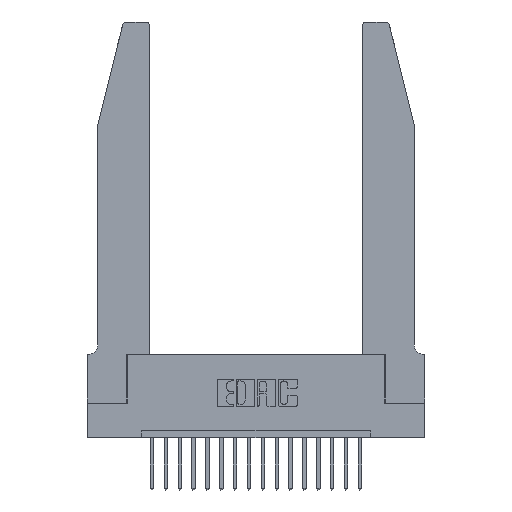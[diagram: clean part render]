
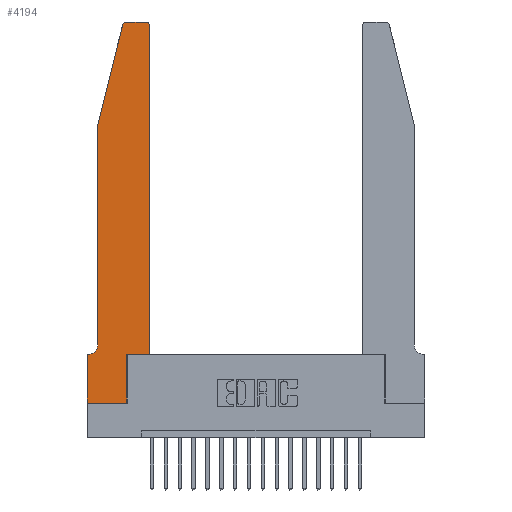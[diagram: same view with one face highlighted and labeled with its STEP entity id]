
A CAD part, top view. The second image highlights one B-rep face of the part: STEP entity #4194.
In plain terms, the highlighted planar face has unit normal (0, 0, 1).
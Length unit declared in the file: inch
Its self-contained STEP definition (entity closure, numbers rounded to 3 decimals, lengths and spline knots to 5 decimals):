
#94 = VERTEX_POINT ( 'NONE', #13322 ) ;
#170 = VERTEX_POINT ( 'NONE', #18015 ) ;
#202 = EDGE_CURVE ( 'NONE', #3944, #170, #8114, .T. ) ;
#376 = DIRECTION ( 'NONE',  ( 1., 0., 0. ) ) ;
#534 = EDGE_CURVE ( 'NONE', #94, #1270, #5633, .T. ) ;
#641 = CARTESIAN_POINT ( 'NONE',  ( 0.2605, 2.75, 0.37 ) ) ;
#1007 = DIRECTION ( 'NONE',  ( -1., 0., 0. ) ) ;
#1154 = CARTESIAN_POINT ( 'NONE',  ( 0.0055, 0.42, 0.37 ) ) ;
#1270 = VERTEX_POINT ( 'NONE', #15781 ) ;
#1276 = CARTESIAN_POINT ( 'NONE',  ( 0., 0.35, 0.37 ) ) ;
#1709 = VECTOR ( 'NONE', #8410, 39.37008 ) ;
#2233 = VERTEX_POINT ( 'NONE', #10709 ) ;
#2391 = ORIENTED_EDGE ( 'NONE', *, *, #17332, .T. ) ;
#2839 = DIRECTION ( 'NONE',  ( 1., 0., 0. ) ) ;
#2897 = DIRECTION ( 'NONE',  ( 0., -1., 0. ) ) ;
#2994 = VERTEX_POINT ( 'NONE', #13306 ) ;
#3384 = VECTOR ( 'NONE', #2897, 39.37008 ) ;
#3480 = CARTESIAN_POINT ( 'NONE',  ( 0., 0., 0.37 ) ) ;
#3659 = CARTESIAN_POINT ( 'NONE',  ( 0.4505, 0.35, 0.37 ) ) ;
#3829 = DIRECTION ( 'NONE',  ( -1., 0., 0. ) ) ;
#3839 = DIRECTION ( 'NONE',  ( -0.239, -0.971, 0. ) ) ;
#3944 = VERTEX_POINT ( 'NONE', #16292 ) ;
#4049 = FACE_OUTER_BOUND ( 'NONE', #19425, .T. ) ;
#4194 = ADVANCED_FACE ( 'NONE', ( #4049 ), #17205, .T. ) ;
#4573 = VERTEX_POINT ( 'NONE', #1276 ) ;
#4658 = LINE ( 'NONE', #12014, #15701 ) ;
#4729 = ORIENTED_EDGE ( 'NONE', *, *, #11184, .T. ) ;
#4768 = ORIENTED_EDGE ( 'NONE', *, *, #5936, .T. ) ;
#4908 = VECTOR ( 'NONE', #3839, 39.37008 ) ;
#5247 = ORIENTED_EDGE ( 'NONE', *, *, #202, .T. ) ;
#5402 = DIRECTION ( 'NONE',  ( -1., 0., 0. ) ) ;
#5448 = AXIS2_PLACEMENT_3D ( 'NONE', #1154, #12026, #1007 ) ;
#5456 = CARTESIAN_POINT ( 'NONE',  ( 0.4505, 0.35, 0.37 ) ) ;
#5633 = CIRCLE ( 'NONE', #6486, 0.03 ) ;
#5805 = ORIENTED_EDGE ( 'NONE', *, *, #534, .T. ) ;
#5936 = EDGE_CURVE ( 'NONE', #16654, #6398, #16736, .T. ) ;
#6065 = CARTESIAN_POINT ( 'NONE',  ( 0.0755, 2., 0.37 ) ) ;
#6201 = ORIENTED_EDGE ( 'NONE', *, *, #19285, .T. ) ;
#6398 = VERTEX_POINT ( 'NONE', #19903 ) ;
#6486 = AXIS2_PLACEMENT_3D ( 'NONE', #19861, #7242, #10382 ) ;
#6542 = AXIS2_PLACEMENT_3D ( 'NONE', #12942, #14470, #376 ) ;
#6652 = LINE ( 'NONE', #13153, #4908 ) ;
#7002 = LINE ( 'NONE', #641, #7955 ) ;
#7242 = DIRECTION ( 'NONE',  ( 0., 0., 1. ) ) ;
#7265 = ORIENTED_EDGE ( 'NONE', *, *, #16557, .T. ) ;
#7582 = LINE ( 'NONE', #11657, #16384 ) ;
#7955 = VECTOR ( 'NONE', #5402, 39.37008 ) ;
#8114 = LINE ( 'NONE', #18491, #17631 ) ;
#8335 = DIRECTION ( 'NONE',  ( 0., 1., 0. ) ) ;
#8339 = ORIENTED_EDGE ( 'NONE', *, *, #18361, .T. ) ;
#8410 = DIRECTION ( 'NONE',  ( 1., 0., 0. ) ) ;
#9039 = LINE ( 'NONE', #6065, #3384 ) ;
#9347 = DIRECTION ( 'NONE',  ( 0., 0., 1. ) ) ;
#9499 = VERTEX_POINT ( 'NONE', #18136 ) ;
#10382 = DIRECTION ( 'NONE',  ( 1., 0., 0. ) ) ;
#10709 = CARTESIAN_POINT ( 'NONE',  ( 0.284, 2.75, 0.37 ) ) ;
#11184 = EDGE_CURVE ( 'NONE', #2994, #9499, #6652, .T. ) ;
#11384 = ORIENTED_EDGE ( 'NONE', *, *, #15175, .T. ) ;
#11543 = LINE ( 'NONE', #3480, #12003 ) ;
#11635 = CARTESIAN_POINT ( 'NONE',  ( 0.0755, 0.42, 0.37 ) ) ;
#11657 = CARTESIAN_POINT ( 'NONE',  ( 0.0755, 0.35, 0.37 ) ) ;
#11877 = ORIENTED_EDGE ( 'NONE', *, *, #19243, .T. ) ;
#12003 = VECTOR ( 'NONE', #18964, 39.37008 ) ;
#12014 = CARTESIAN_POINT ( 'NONE',  ( 0.2865, 0.35, 0.37 ) ) ;
#12026 = DIRECTION ( 'NONE',  ( 0., 0., -1. ) ) ;
#12210 = ORIENTED_EDGE ( 'NONE', *, *, #19889, .T. ) ;
#12246 = CIRCLE ( 'NONE', #6542, 0.03 ) ;
#12252 = CARTESIAN_POINT ( 'NONE',  ( 0., 0.35, 0.37 ) ) ;
#12616 = EDGE_CURVE ( 'NONE', #9499, #16654, #9039, .T. ) ;
#12942 = CARTESIAN_POINT ( 'NONE',  ( 0.284, 2.72, 0.37 ) ) ;
#13031 = LINE ( 'NONE', #3659, #14016 ) ;
#13153 = CARTESIAN_POINT ( 'NONE',  ( 0.0755, 2., 0.37 ) ) ;
#13306 = CARTESIAN_POINT ( 'NONE',  ( 0.25487, 2.72718, 0.37 ) ) ;
#13322 = CARTESIAN_POINT ( 'NONE',  ( 0.4505, 2.72, 0.37 ) ) ;
#13426 = CARTESIAN_POINT ( 'NONE',  ( 0.2865, 0.35, 0.37 ) ) ;
#13821 = VERTEX_POINT ( 'NONE', #13426 ) ;
#14016 = VECTOR ( 'NONE', #8335, 39.37008 ) ;
#14086 = AXIS2_PLACEMENT_3D ( 'NONE', #12252, #9347, #2839 ) ;
#14154 = ORIENTED_EDGE ( 'NONE', *, *, #12616, .T. ) ;
#14218 = CARTESIAN_POINT ( 'NONE',  ( 0.4505, 0.35, 0.37 ) ) ;
#14470 = DIRECTION ( 'NONE',  ( 0., 0., 1. ) ) ;
#14499 = LINE ( 'NONE', #5456, #1709 ) ;
#15175 = EDGE_CURVE ( 'NONE', #1270, #2233, #7002, .T. ) ;
#15701 = VECTOR ( 'NONE', #19988, 39.37008 ) ;
#15781 = CARTESIAN_POINT ( 'NONE',  ( 0.4205, 2.75, 0.37 ) ) ;
#16292 = CARTESIAN_POINT ( 'NONE',  ( 0., 0., 0.37 ) ) ;
#16384 = VECTOR ( 'NONE', #3829, 39.37008 ) ;
#16557 = EDGE_CURVE ( 'NONE', #20300, #94, #13031, .T. ) ;
#16654 = VERTEX_POINT ( 'NONE', #11635 ) ;
#16736 = CIRCLE ( 'NONE', #5448, 0.07 ) ;
#17205 = PLANE ( 'NONE',  #14086 ) ;
#17332 = EDGE_CURVE ( 'NONE', #170, #13821, #4658, .T. ) ;
#17631 = VECTOR ( 'NONE', #20080, 39.37008 ) ;
#18015 = CARTESIAN_POINT ( 'NONE',  ( 0.2865, 0., 0.37 ) ) ;
#18136 = CARTESIAN_POINT ( 'NONE',  ( 0.0755, 2., 0.37 ) ) ;
#18361 = EDGE_CURVE ( 'NONE', #13821, #20300, #14499, .T. ) ;
#18491 = CARTESIAN_POINT ( 'NONE',  ( 0., 0., 0.37 ) ) ;
#18964 = DIRECTION ( 'NONE',  ( 0., -1., 0. ) ) ;
#19243 = EDGE_CURVE ( 'NONE', #4573, #3944, #11543, .T. ) ;
#19285 = EDGE_CURVE ( 'NONE', #2233, #2994, #12246, .T. ) ;
#19425 = EDGE_LOOP ( 'NONE', ( #11384, #6201, #4729, #14154, #4768, #12210, #11877, #5247, #2391, #8339, #7265, #5805 ) ) ;
#19861 = CARTESIAN_POINT ( 'NONE',  ( 0.4205, 2.72, 0.37 ) ) ;
#19889 = EDGE_CURVE ( 'NONE', #6398, #4573, #7582, .T. ) ;
#19903 = CARTESIAN_POINT ( 'NONE',  ( 0.0055, 0.35, 0.37 ) ) ;
#19988 = DIRECTION ( 'NONE',  ( 0., 1., 0. ) ) ;
#20080 = DIRECTION ( 'NONE',  ( 1., 0., 0. ) ) ;
#20300 = VERTEX_POINT ( 'NONE', #14218 ) ;
